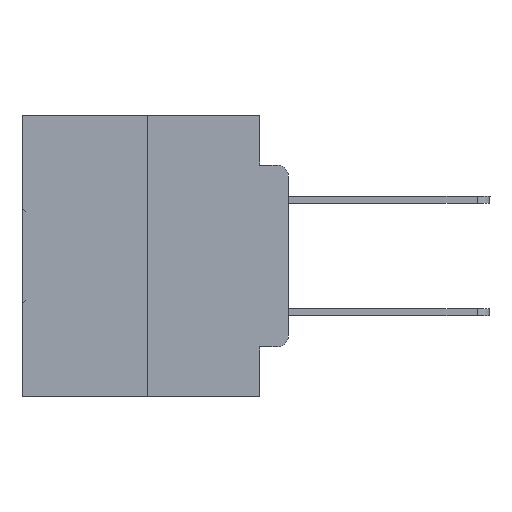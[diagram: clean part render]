
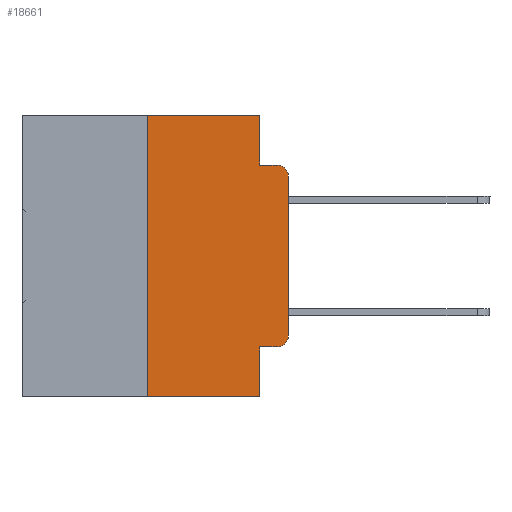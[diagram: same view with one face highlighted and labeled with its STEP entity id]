
A CAD part, left-side view. The second image highlights one B-rep face of the part: STEP entity #18661.
In plain terms, the highlighted planar face has unit normal (-1, 0, 0).
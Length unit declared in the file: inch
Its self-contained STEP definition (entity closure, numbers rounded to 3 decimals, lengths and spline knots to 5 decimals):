
#32 = CARTESIAN_POINT ( 'NONE',  ( 0., 0.25, 0. ) ) ;
#39 = CARTESIAN_POINT ( 'NONE',  ( 0., 0.051, 0. ) ) ;
#162 = EDGE_CURVE ( 'NONE', #437, #11612, #25931, .T. ) ;
#437 = VERTEX_POINT ( 'NONE', #32 ) ;
#470 = FACE_OUTER_BOUND ( 'NONE', #5013, .T. ) ;
#663 = DIRECTION ( 'NONE',  ( 0., 0., -1. ) ) ;
#732 = VECTOR ( 'NONE', #30168, 39.37008 ) ;
#1015 = VERTEX_POINT ( 'NONE', #30427 ) ;
#1032 = CARTESIAN_POINT ( 'NONE',  ( 0., 0., 0. ) ) ;
#1287 = VECTOR ( 'NONE', #17335, 39.37008 ) ;
#1335 = AXIS2_PLACEMENT_3D ( 'NONE', #3134, #16418, #663 ) ;
#1557 = DIRECTION ( 'NONE',  ( 0., -1., 0. ) ) ;
#1586 = ORIENTED_EDGE ( 'NONE', *, *, #19409, .T. ) ;
#2409 = ORIENTED_EDGE ( 'NONE', *, *, #162, .F. ) ;
#2484 = CARTESIAN_POINT ( 'NONE',  ( 0., 0.051, -0.4115 ) ) ;
#2597 = EDGE_CURVE ( 'NONE', #9192, #7681, #19618, .T. ) ;
#3134 = CARTESIAN_POINT ( 'NONE',  ( 0., 0.473, 0. ) ) ;
#3672 = CARTESIAN_POINT ( 'NONE',  ( 0., 0.051, -0.5 ) ) ;
#3927 = CARTESIAN_POINT ( 'NONE',  ( 0., 0., -0.1085 ) ) ;
#4423 = EDGE_CURVE ( 'NONE', #30329, #437, #21179, .T. ) ;
#4752 = VECTOR ( 'NONE', #1557, 39.37008 ) ;
#5013 = EDGE_LOOP ( 'NONE', ( #16731, #13791, #13762, #12224, #2409, #21849, #1586, #23394, #15194, #31449 ) ) ;
#5528 = CARTESIAN_POINT ( 'NONE',  ( 0., 0.473, 0. ) ) ;
#6696 = VECTOR ( 'NONE', #10776, 39.37008 ) ;
#6705 = VECTOR ( 'NONE', #20641, 39.37008 ) ;
#7329 = CARTESIAN_POINT ( 'NONE',  ( 0., 0.051, -0.0885 ) ) ;
#7681 = VERTEX_POINT ( 'NONE', #3672 ) ;
#7949 = EDGE_CURVE ( 'NONE', #11612, #1015, #31426, .T. ) ;
#8113 = CARTESIAN_POINT ( 'NONE',  ( 0., 0.25, -0.5 ) ) ;
#8646 = CARTESIAN_POINT ( 'NONE',  ( 0., 0.02, -0.3915 ) ) ;
#9192 = VERTEX_POINT ( 'NONE', #11218 ) ;
#9722 = EDGE_CURVE ( 'NONE', #30570, #19080, #10029, .T. ) ;
#10029 = CIRCLE ( 'NONE', #25309, 0.02 ) ;
#10514 = DIRECTION ( 'NONE',  ( -1., 0., 0. ) ) ;
#10776 = DIRECTION ( 'NONE',  ( 0., 0., -1. ) ) ;
#10916 = CARTESIAN_POINT ( 'NONE',  ( 0., 0.051, 0. ) ) ;
#11218 = CARTESIAN_POINT ( 'NONE',  ( 0., 0.051, -0.4115 ) ) ;
#11258 = DIRECTION ( 'NONE',  ( 0., 0., -1. ) ) ;
#11424 = EDGE_CURVE ( 'NONE', #1015, #19080, #23795, .T. ) ;
#11612 = VERTEX_POINT ( 'NONE', #39 ) ;
#12224 = ORIENTED_EDGE ( 'NONE', *, *, #7949, .F. ) ;
#13252 = VECTOR ( 'NONE', #19380, 39.37008 ) ;
#13762 = ORIENTED_EDGE ( 'NONE', *, *, #11424, .F. ) ;
#13791 = ORIENTED_EDGE ( 'NONE', *, *, #9722, .T. ) ;
#14950 = EDGE_CURVE ( 'NONE', #28806, #30570, #20527, .T. ) ;
#15194 = ORIENTED_EDGE ( 'NONE', *, *, #27930, .T. ) ;
#15262 = DIRECTION ( 'NONE',  ( 0., 0., -1. ) ) ;
#16418 = DIRECTION ( 'NONE',  ( 1., 0., 0. ) ) ;
#16731 = ORIENTED_EDGE ( 'NONE', *, *, #14950, .T. ) ;
#16763 = DIRECTION ( 'NONE',  ( 0., 0., 1. ) ) ;
#17191 = VERTEX_POINT ( 'NONE', #28556 ) ;
#17335 = DIRECTION ( 'NONE',  ( 0., 0., 1. ) ) ;
#17430 = CARTESIAN_POINT ( 'NONE',  ( 0., 0.25, 0. ) ) ;
#17704 = CARTESIAN_POINT ( 'NONE',  ( 0., 0.051, 0. ) ) ;
#18242 = VECTOR ( 'NONE', #15262, 39.37008 ) ;
#18661 = ADVANCED_FACE ( 'NONE', ( #470 ), #23841, .F. ) ;
#18840 = LINE ( 'NONE', #2484, #6705 ) ;
#19080 = VERTEX_POINT ( 'NONE', #33044 ) ;
#19262 = LINE ( 'NONE', #26766, #13252 ) ;
#19297 = CARTESIAN_POINT ( 'NONE',  ( 0., 0., -0.3915 ) ) ;
#19380 = DIRECTION ( 'NONE',  ( 0., -1., 0. ) ) ;
#19409 = EDGE_CURVE ( 'NONE', #30329, #7681, #19262, .T. ) ;
#19618 = LINE ( 'NONE', #10916, #6696 ) ;
#20037 = AXIS2_PLACEMENT_3D ( 'NONE', #8646, #26406, #11258 ) ;
#20527 = LINE ( 'NONE', #1032, #26344 ) ;
#20641 = DIRECTION ( 'NONE',  ( 0., -1., 0. ) ) ;
#21179 = LINE ( 'NONE', #17430, #1287 ) ;
#21849 = ORIENTED_EDGE ( 'NONE', *, *, #4423, .F. ) ;
#23394 = ORIENTED_EDGE ( 'NONE', *, *, #2597, .F. ) ;
#23795 = LINE ( 'NONE', #7329, #732 ) ;
#23841 = PLANE ( 'NONE',  #1335 ) ;
#25309 = AXIS2_PLACEMENT_3D ( 'NONE', #25684, #10514, #28183 ) ;
#25684 = CARTESIAN_POINT ( 'NONE',  ( 0., 0.02, -0.1085 ) ) ;
#25931 = LINE ( 'NONE', #5528, #4752 ) ;
#26247 = EDGE_CURVE ( 'NONE', #17191, #28806, #28601, .T. ) ;
#26344 = VECTOR ( 'NONE', #16763, 39.37008 ) ;
#26406 = DIRECTION ( 'NONE',  ( -1., 0., 0. ) ) ;
#26766 = CARTESIAN_POINT ( 'NONE',  ( 0., 0.473, -0.5 ) ) ;
#27930 = EDGE_CURVE ( 'NONE', #9192, #17191, #18840, .T. ) ;
#28183 = DIRECTION ( 'NONE',  ( 0., 0., -1. ) ) ;
#28556 = CARTESIAN_POINT ( 'NONE',  ( 0., 0.02, -0.4115 ) ) ;
#28601 = CIRCLE ( 'NONE', #20037, 0.02 ) ;
#28806 = VERTEX_POINT ( 'NONE', #19297 ) ;
#30168 = DIRECTION ( 'NONE',  ( 0., -1., 0. ) ) ;
#30329 = VERTEX_POINT ( 'NONE', #8113 ) ;
#30427 = CARTESIAN_POINT ( 'NONE',  ( 0., 0.051, -0.0885 ) ) ;
#30570 = VERTEX_POINT ( 'NONE', #3927 ) ;
#31426 = LINE ( 'NONE', #17704, #18242 ) ;
#31449 = ORIENTED_EDGE ( 'NONE', *, *, #26247, .T. ) ;
#33044 = CARTESIAN_POINT ( 'NONE',  ( 0., 0.02, -0.0885 ) ) ;
